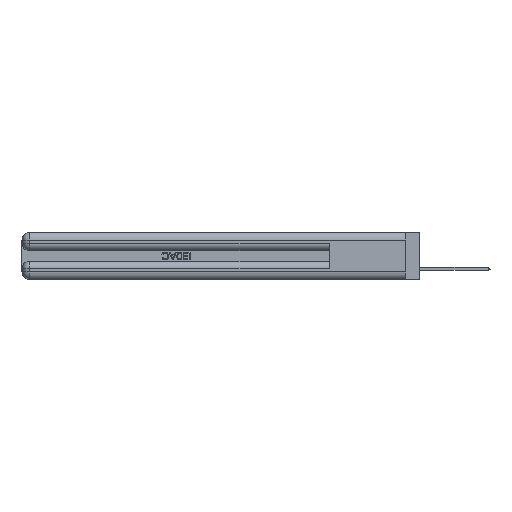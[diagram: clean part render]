
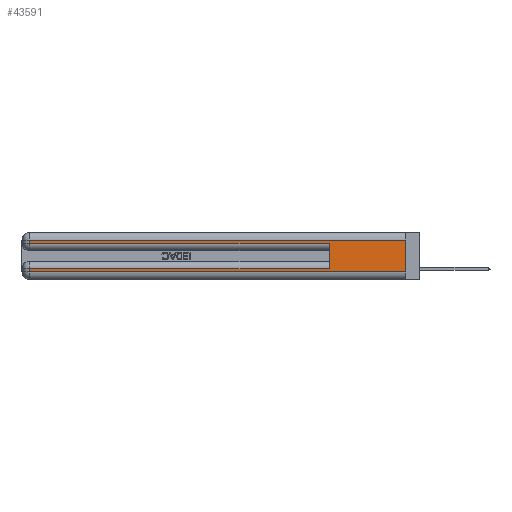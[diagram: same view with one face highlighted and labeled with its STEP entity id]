
A CAD part, left-side view. The second image highlights one B-rep face of the part: STEP entity #43591.
In plain terms, the highlighted planar face has unit normal (-1, 0, 0).
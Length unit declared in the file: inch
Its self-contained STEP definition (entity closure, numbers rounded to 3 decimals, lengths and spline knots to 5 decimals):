
#745 = VERTEX_POINT ( 'NONE', #11750 ) ;
#1895 = EDGE_LOOP ( 'NONE', ( #44239, #51005, #35711, #38078, #51206, #9153, #16737, #42521 ) ) ;
#1896 = CARTESIAN_POINT ( 'NONE',  ( 0., 0., 0.285 ) ) ;
#1981 = VERTEX_POINT ( 'NONE', #8640 ) ;
#2088 = DIRECTION ( 'NONE',  ( 0., 0., -1. ) ) ;
#3375 = EDGE_CURVE ( 'NONE', #11034, #1981, #52178, .T. ) ;
#3451 = EDGE_CURVE ( 'NONE', #1981, #745, #27796, .T. ) ;
#4683 = LINE ( 'NONE', #36887, #9785 ) ;
#4816 = VERTEX_POINT ( 'NONE', #23754 ) ;
#5775 = DIRECTION ( 'NONE',  ( 0., -1., 0. ) ) ;
#5820 = DIRECTION ( 'NONE',  ( 1., 0., 0. ) ) ;
#8640 = CARTESIAN_POINT ( 'NONE',  ( 0., 2.94, 0.285 ) ) ;
#9153 = ORIENTED_EDGE ( 'NONE', *, *, #11798, .T. ) ;
#9785 = VECTOR ( 'NONE', #20219, 39.37008 ) ;
#10053 = FACE_OUTER_BOUND ( 'NONE', #1895, .T. ) ;
#11034 = VERTEX_POINT ( 'NONE', #14424 ) ;
#11750 = CARTESIAN_POINT ( 'NONE',  ( 0., 0.6, 0.285 ) ) ;
#11798 = EDGE_CURVE ( 'NONE', #30262, #4816, #12441, .T. ) ;
#12300 = DIRECTION ( 'NONE',  ( 0., 0., 1. ) ) ;
#12441 = LINE ( 'NONE', #51980, #47729 ) ;
#13666 = LINE ( 'NONE', #17516, #38665 ) ;
#14424 = CARTESIAN_POINT ( 'NONE',  ( 0., 2.94, 0.31 ) ) ;
#14509 = CARTESIAN_POINT ( 'NONE',  ( 0., 2.94, 0.06 ) ) ;
#16737 = ORIENTED_EDGE ( 'NONE', *, *, #45833, .T. ) ;
#17516 = CARTESIAN_POINT ( 'NONE',  ( 0., 2.94, 0.37 ) ) ;
#18861 = VECTOR ( 'NONE', #2088, 39.37008 ) ;
#20219 = DIRECTION ( 'NONE',  ( 0., 1., 0. ) ) ;
#20742 = AXIS2_PLACEMENT_3D ( 'NONE', #38360, #5820, #42668 ) ;
#21395 = VECTOR ( 'NONE', #5775, 39.37008 ) ;
#22134 = DIRECTION ( 'NONE',  ( 0., 0., -1. ) ) ;
#22456 = CARTESIAN_POINT ( 'NONE',  ( 0., 0., 0.06 ) ) ;
#22745 = LINE ( 'NONE', #46763, #21395 ) ;
#23754 = CARTESIAN_POINT ( 'NONE',  ( 0., 2.94, 0.085 ) ) ;
#26204 = DIRECTION ( 'NONE',  ( 0., 0., -1. ) ) ;
#26580 = CARTESIAN_POINT ( 'NONE',  ( 0., 0., 0.37 ) ) ;
#27145 = DIRECTION ( 'NONE',  ( 0., -1., 0. ) ) ;
#27796 = LINE ( 'NONE', #1896, #37318 ) ;
#29561 = VECTOR ( 'NONE', #26204, 39.37008 ) ;
#30262 = VERTEX_POINT ( 'NONE', #37341 ) ;
#33601 = LINE ( 'NONE', #34875, #36830 ) ;
#34084 = PLANE ( 'NONE',  #20742 ) ;
#34875 = CARTESIAN_POINT ( 'NONE',  ( 0., 0.6, 0.145 ) ) ;
#35056 = VERTEX_POINT ( 'NONE', #38827 ) ;
#35552 = EDGE_CURVE ( 'NONE', #49868, #44947, #22745, .T. ) ;
#35711 = ORIENTED_EDGE ( 'NONE', *, *, #3375, .T. ) ;
#36187 = DIRECTION ( 'NONE',  ( 0., 1., 0. ) ) ;
#36254 = EDGE_CURVE ( 'NONE', #30262, #745, #33601, .T. ) ;
#36830 = VECTOR ( 'NONE', #12300, 39.37008 ) ;
#36887 = CARTESIAN_POINT ( 'NONE',  ( 0., 0., 0.31 ) ) ;
#37318 = VECTOR ( 'NONE', #27145, 39.37008 ) ;
#37341 = CARTESIAN_POINT ( 'NONE',  ( 0., 0.6, 0.085 ) ) ;
#38078 = ORIENTED_EDGE ( 'NONE', *, *, #3451, .T. ) ;
#38360 = CARTESIAN_POINT ( 'NONE',  ( 0., 0., 0.37 ) ) ;
#38665 = VECTOR ( 'NONE', #22134, 39.37008 ) ;
#38827 = CARTESIAN_POINT ( 'NONE',  ( 0., 0., 0.31 ) ) ;
#42521 = ORIENTED_EDGE ( 'NONE', *, *, #35552, .T. ) ;
#42668 = DIRECTION ( 'NONE',  ( 0., 0., -1. ) ) ;
#43591 = ADVANCED_FACE ( 'NONE', ( #10053 ), #34084, .F. ) ;
#44239 = ORIENTED_EDGE ( 'NONE', *, *, #45452, .F. ) ;
#44947 = VERTEX_POINT ( 'NONE', #22456 ) ;
#45452 = EDGE_CURVE ( 'NONE', #35056, #44947, #50203, .T. ) ;
#45833 = EDGE_CURVE ( 'NONE', #4816, #49868, #13666, .T. ) ;
#46277 = EDGE_CURVE ( 'NONE', #35056, #11034, #4683, .T. ) ;
#46435 = CARTESIAN_POINT ( 'NONE',  ( 0., 2.94, 0.37 ) ) ;
#46763 = CARTESIAN_POINT ( 'NONE',  ( 0., 0., 0.06 ) ) ;
#47729 = VECTOR ( 'NONE', #36187, 39.37008 ) ;
#49868 = VERTEX_POINT ( 'NONE', #14509 ) ;
#50203 = LINE ( 'NONE', #26580, #18861 ) ;
#51005 = ORIENTED_EDGE ( 'NONE', *, *, #46277, .T. ) ;
#51206 = ORIENTED_EDGE ( 'NONE', *, *, #36254, .F. ) ;
#51980 = CARTESIAN_POINT ( 'NONE',  ( 0., 0., 0.085 ) ) ;
#52178 = LINE ( 'NONE', #46435, #29561 ) ;
